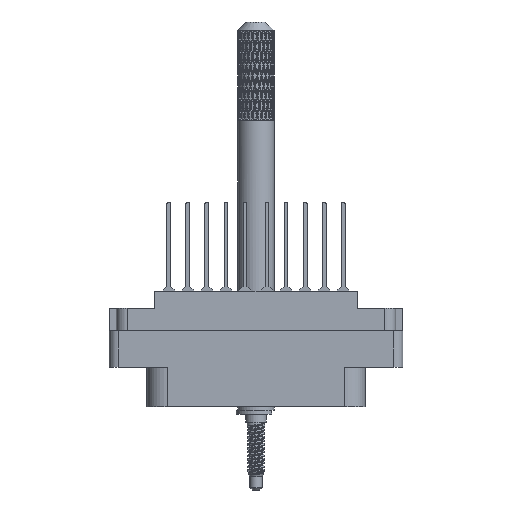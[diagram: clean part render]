
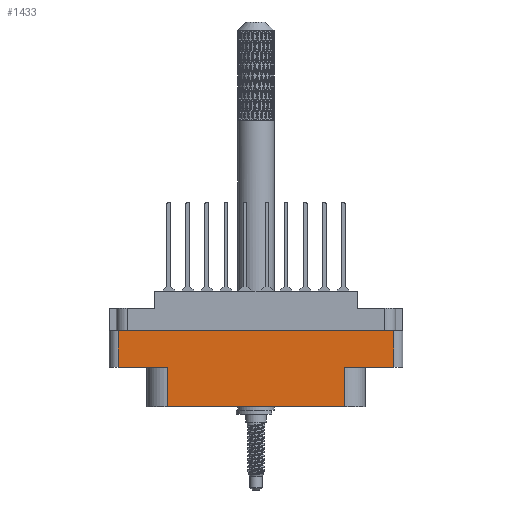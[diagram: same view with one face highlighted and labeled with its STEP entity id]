
A CAD part, front view. The second image highlights one B-rep face of the part: STEP entity #1433.
In plain terms, the highlighted planar face has unit normal (0, -1, 0).
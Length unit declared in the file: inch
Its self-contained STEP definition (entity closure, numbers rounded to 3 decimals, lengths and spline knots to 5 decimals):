
#1433 = ADVANCED_FACE ( 'NONE', ( #78184 ), #10818, .T. ) ;
#1741 = ORIENTED_EDGE ( 'NONE', *, *, #97314, .T. ) ;
#2583 = EDGE_CURVE ( 'NONE', #28088, #67343, #74289, .T. ) ;
#3120 = CARTESIAN_POINT ( 'NONE',  ( 0.604, -0.438, -0.52 ) ) ;
#3311 = DIRECTION ( 'NONE',  ( 0., 0., -1. ) ) ;
#5272 = VERTEX_POINT ( 'NONE', #103500 ) ;
#10359 = VERTEX_POINT ( 'NONE', #39779 ) ;
#10756 = EDGE_CURVE ( 'NONE', #67343, #10359, #41738, .T. ) ;
#10818 = PLANE ( 'NONE',  #53163 ) ;
#11158 = CARTESIAN_POINT ( 'NONE',  ( -1., -0.438, -0.789 ) ) ;
#12314 = VECTOR ( 'NONE', #3311, 39.37008 ) ;
#14412 = VECTOR ( 'NONE', #37407, 39.37008 ) ;
#15026 = VERTEX_POINT ( 'NONE', #52559 ) ;
#15373 = CARTESIAN_POINT ( 'NONE',  ( 0.604, -0.438, -0.52 ) ) ;
#16787 = VECTOR ( 'NONE', #38597, 39.37008 ) ;
#18458 = LINE ( 'NONE', #98189, #12314 ) ;
#18567 = CARTESIAN_POINT ( 'NONE',  ( -0.604, -0.438, -0.789 ) ) ;
#19447 = LINE ( 'NONE', #100430, #26916 ) ;
#23806 = VECTOR ( 'NONE', #57623, 39.37008 ) ;
#25610 = EDGE_CURVE ( 'NONE', #81060, #5272, #19447, .T. ) ;
#26916 = VECTOR ( 'NONE', #69439, 39.37008 ) ;
#26963 = VECTOR ( 'NONE', #68499, 39.37008 ) ;
#27647 = CARTESIAN_POINT ( 'NONE',  ( -0.938, -0.438, -0.789 ) ) ;
#28041 = CARTESIAN_POINT ( 'NONE',  ( 0.938, -0.438, -0.789 ) ) ;
#28088 = VERTEX_POINT ( 'NONE', #51965 ) ;
#29391 = ORIENTED_EDGE ( 'NONE', *, *, #32547, .T. ) ;
#30539 = CARTESIAN_POINT ( 'NONE',  ( 0., -0.438, -0.52 ) ) ;
#31753 = ORIENTED_EDGE ( 'NONE', *, *, #82990, .F. ) ;
#32547 = EDGE_CURVE ( 'NONE', #5272, #98101, #81191, .T. ) ;
#35185 = ORIENTED_EDGE ( 'NONE', *, *, #2583, .T. ) ;
#37407 = DIRECTION ( 'NONE',  ( 0., 0., -1. ) ) ;
#38597 = DIRECTION ( 'NONE',  ( 1., 0., 0. ) ) ;
#39779 = CARTESIAN_POINT ( 'NONE',  ( -0.604, -0.438, -0.52 ) ) ;
#41738 = LINE ( 'NONE', #30539, #16787 ) ;
#43738 = CARTESIAN_POINT ( 'NONE',  ( 0., -0.438, -0.52 ) ) ;
#45630 = LINE ( 'NONE', #47780, #88035 ) ;
#47780 = CARTESIAN_POINT ( 'NONE',  ( 0., -0.438, -0.268 ) ) ;
#50620 = DIRECTION ( 'NONE',  ( 0., 0., -1. ) ) ;
#51965 = CARTESIAN_POINT ( 'NONE',  ( -0.938, -0.438, -0.268 ) ) ;
#52559 = CARTESIAN_POINT ( 'NONE',  ( 0.938, -0.438, -0.268 ) ) ;
#53163 = AXIS2_PLACEMENT_3D ( 'NONE', #11158, #73973, #50620 ) ;
#57623 = DIRECTION ( 'NONE',  ( 0., 0., 1. ) ) ;
#59630 = CARTESIAN_POINT ( 'NONE',  ( 0.938, -0.438, -0.52 ) ) ;
#60579 = DIRECTION ( 'NONE',  ( 0., 0., 1. ) ) ;
#61859 = VERTEX_POINT ( 'NONE', #59630 ) ;
#66586 = EDGE_LOOP ( 'NONE', ( #31753, #35185, #82224, #1741, #68930, #29391, #90509, #78621 ) ) ;
#67343 = VERTEX_POINT ( 'NONE', #101238 ) ;
#68499 = DIRECTION ( 'NONE',  ( -1., 0., 0. ) ) ;
#68930 = ORIENTED_EDGE ( 'NONE', *, *, #25610, .T. ) ;
#69439 = DIRECTION ( 'NONE',  ( 1., 0., 0. ) ) ;
#73973 = DIRECTION ( 'NONE',  ( 0., -1., 0. ) ) ;
#74289 = LINE ( 'NONE', #27647, #14412 ) ;
#78184 = FACE_OUTER_BOUND ( 'NONE', #66586, .T. ) ;
#78476 = DIRECTION ( 'NONE',  ( 1., 0., 0. ) ) ;
#78621 = ORIENTED_EDGE ( 'NONE', *, *, #97636, .T. ) ;
#81060 = VERTEX_POINT ( 'NONE', #18567 ) ;
#81191 = LINE ( 'NONE', #3120, #23806 ) ;
#82224 = ORIENTED_EDGE ( 'NONE', *, *, #10756, .T. ) ;
#82990 = EDGE_CURVE ( 'NONE', #28088, #15026, #45630, .T. ) ;
#88035 = VECTOR ( 'NONE', #78476, 39.37008 ) ;
#90509 = ORIENTED_EDGE ( 'NONE', *, *, #99168, .F. ) ;
#92108 = VECTOR ( 'NONE', #60579, 39.37008 ) ;
#97314 = EDGE_CURVE ( 'NONE', #10359, #81060, #18458, .T. ) ;
#97636 = EDGE_CURVE ( 'NONE', #61859, #15026, #98329, .T. ) ;
#98101 = VERTEX_POINT ( 'NONE', #15373 ) ;
#98148 = LINE ( 'NONE', #43738, #26963 ) ;
#98189 = CARTESIAN_POINT ( 'NONE',  ( -0.604, -0.438, -0.789 ) ) ;
#98329 = LINE ( 'NONE', #28041, #92108 ) ;
#99168 = EDGE_CURVE ( 'NONE', #61859, #98101, #98148, .T. ) ;
#100430 = CARTESIAN_POINT ( 'NONE',  ( -1., -0.438, -0.789 ) ) ;
#101238 = CARTESIAN_POINT ( 'NONE',  ( -0.938, -0.438, -0.52 ) ) ;
#103500 = CARTESIAN_POINT ( 'NONE',  ( 0.604, -0.438, -0.789 ) ) ;
